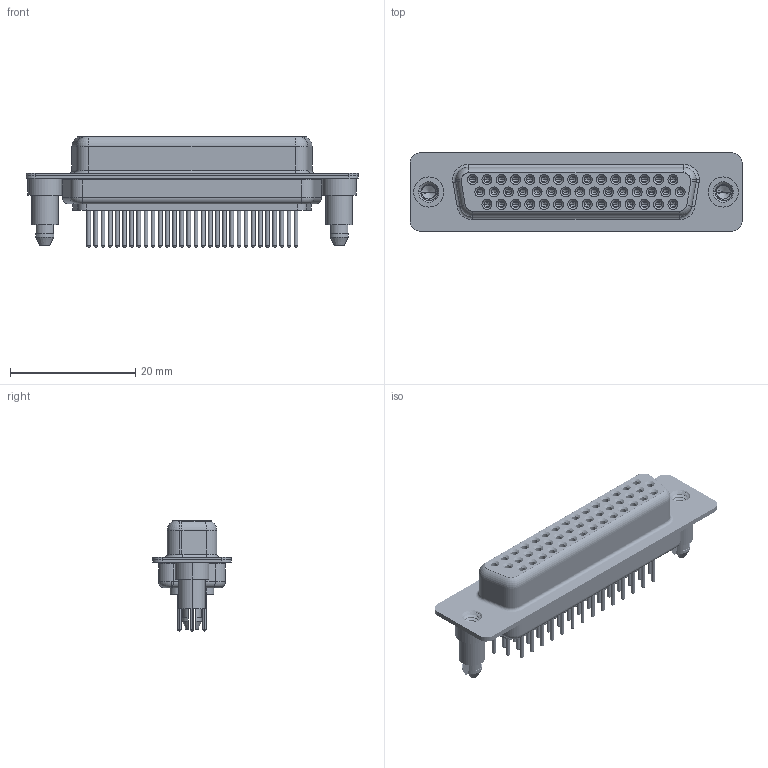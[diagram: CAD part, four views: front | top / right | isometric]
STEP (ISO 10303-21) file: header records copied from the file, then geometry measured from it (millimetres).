
FILE_DESCRIPTION (( 'STEP AP203' ), '1' );
FILE_NAME ('638-M44-230-BT5.STEP', '2022-07-05T20:10:50', ( '' ), ( '' ), 'SwSTEP 2.0', 'SolidWorks 2020', '' );
FILE_SCHEMA (( 'CONFIG_CONTROL_DESIGN' ));
Length unit declared in the file: millimetre
Products named in the file (8): 638-M44-230-BT5; 638M 4-40 Threaded Boardlock; 638M Contact Row 3_30; 638M Contact Row 2_30; 638M Shell Rear_44 Contacts; 638M Shell Front_44 Contacts; 638M Housing_44 Contacts; 638M Contact Row 1_30
Assembly tree (49 placements, depth 2):
  638-M44-230-BT5
    638M Housing_44 Contacts
    638M Shell Front_44 Contacts
    638M Shell Rear_44 Contacts
    638M Contact Row 1_30  x15
    638M Contact Row 2_30  x15
    638M Contact Row 3_30  x14
    638M 4-40 Threaded Boardlock  x2
Bounding box: 53.05 x 12.5 x 17.6 mm (x, y, z)
Volume: 3669.6 mm3; surface area: 12352.2 mm2
Topology: 49 solids, 49 shells, 2749 faces, 6361 edges, 3901 vertices
Faces by surface type: cylinder 1005, plane 743, torus 673, cone 322, bspline 6
Entity records: 31514 total; most frequent: CARTESIAN_POINT 6562, DIRECTION 5359, ORIENTED_EDGE 4376, AXIS2_PLACEMENT_3D 2279, EDGE_CURVE 2188, VERTEX_POINT 1387, CIRCLE 1261, EDGE_LOOP 1223
